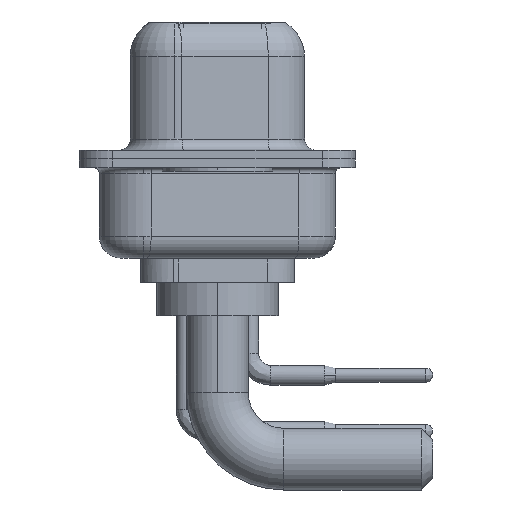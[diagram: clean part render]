
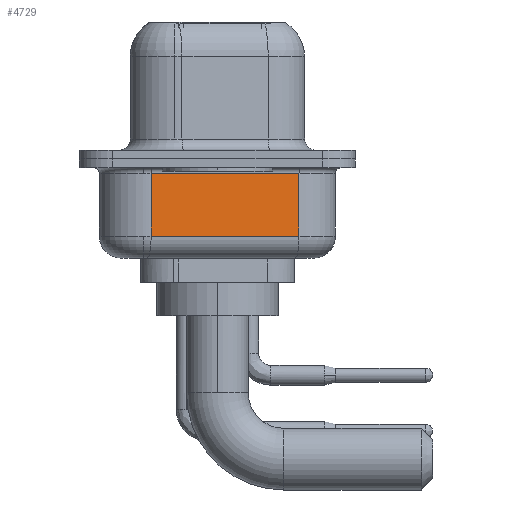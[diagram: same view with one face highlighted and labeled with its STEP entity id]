
A CAD part, left-side view. The second image highlights one B-rep face of the part: STEP entity #4729.
In plain terms, the highlighted planar face has unit normal (-0.985, -0.174, 0).
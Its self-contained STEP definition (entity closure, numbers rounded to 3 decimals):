
#302 = CARTESIAN_POINT ( 'NONE',  ( 4.062, -3.697, -3.5 ) ) ;
#382 = VERTEX_POINT ( 'NONE', #13147 ) ;
#1154 = DIRECTION ( 'NONE',  ( 0.985, 0.174, 0. ) ) ;
#2148 = CARTESIAN_POINT ( 'NONE',  ( 2.88, 3.003, -3.5 ) ) ;
#2941 = DIRECTION ( 'NONE',  ( -0.174, 0.985, 0. ) ) ;
#3416 = ORIENTED_EDGE ( 'NONE', *, *, #13370, .T. ) ;
#4729 = ADVANCED_FACE ( 'NONE', ( #16502 ), #13402, .F. ) ;
#5049 = LINE ( 'NONE', #10281, #5713 ) ;
#5650 = EDGE_CURVE ( 'NONE', #13729, #382, #14908, .T. ) ;
#5713 = VECTOR ( 'NONE', #11848, 1000. ) ;
#5759 = DIRECTION ( 'NONE',  ( 0., 0., 1. ) ) ;
#5966 = LINE ( 'NONE', #19325, #15231 ) ;
#6481 = VERTEX_POINT ( 'NONE', #6691 ) ;
#6691 = CARTESIAN_POINT ( 'NONE',  ( 2.88, 3.003, -0.65 ) ) ;
#7219 = CARTESIAN_POINT ( 'NONE',  ( 2.88, 3.003, -4.5 ) ) ;
#7297 = VERTEX_POINT ( 'NONE', #2148 ) ;
#8168 = CARTESIAN_POINT ( 'NONE',  ( 2.88, 3.003, -4.5 ) ) ;
#9043 = ORIENTED_EDGE ( 'NONE', *, *, #16045, .T. ) ;
#10281 = CARTESIAN_POINT ( 'NONE',  ( 2.88, 3.003, -3.5 ) ) ;
#11003 = LINE ( 'NONE', #7219, #18174 ) ;
#11626 = EDGE_LOOP ( 'NONE', ( #13173, #3416, #21413, #9043 ) ) ;
#11848 = DIRECTION ( 'NONE',  ( 0.174, -0.985, 0. ) ) ;
#13147 = CARTESIAN_POINT ( 'NONE',  ( 4.062, -3.697, -0.65 ) ) ;
#13173 = ORIENTED_EDGE ( 'NONE', *, *, #19162, .F. ) ;
#13241 = DIRECTION ( 'NONE',  ( 0., 0., 1. ) ) ;
#13370 = EDGE_CURVE ( 'NONE', #7297, #13729, #5049, .T. ) ;
#13402 = PLANE ( 'NONE',  #13671 ) ;
#13671 = AXIS2_PLACEMENT_3D ( 'NONE', #8168, #1154, #2941 ) ;
#13729 = VERTEX_POINT ( 'NONE', #302 ) ;
#14058 = VECTOR ( 'NONE', #13241, 1000. ) ;
#14908 = LINE ( 'NONE', #21681, #14058 ) ;
#15231 = VECTOR ( 'NONE', #18087, 1000. ) ;
#16045 = EDGE_CURVE ( 'NONE', #382, #6481, #5966, .T. ) ;
#16502 = FACE_OUTER_BOUND ( 'NONE', #11626, .T. ) ;
#18087 = DIRECTION ( 'NONE',  ( -0.174, 0.985, 0. ) ) ;
#18174 = VECTOR ( 'NONE', #5759, 1000. ) ;
#19162 = EDGE_CURVE ( 'NONE', #7297, #6481, #11003, .T. ) ;
#19325 = CARTESIAN_POINT ( 'NONE',  ( 2.88, 3.003, -0.65 ) ) ;
#21413 = ORIENTED_EDGE ( 'NONE', *, *, #5650, .T. ) ;
#21681 = CARTESIAN_POINT ( 'NONE',  ( 4.062, -3.697, -4.5 ) ) ;
